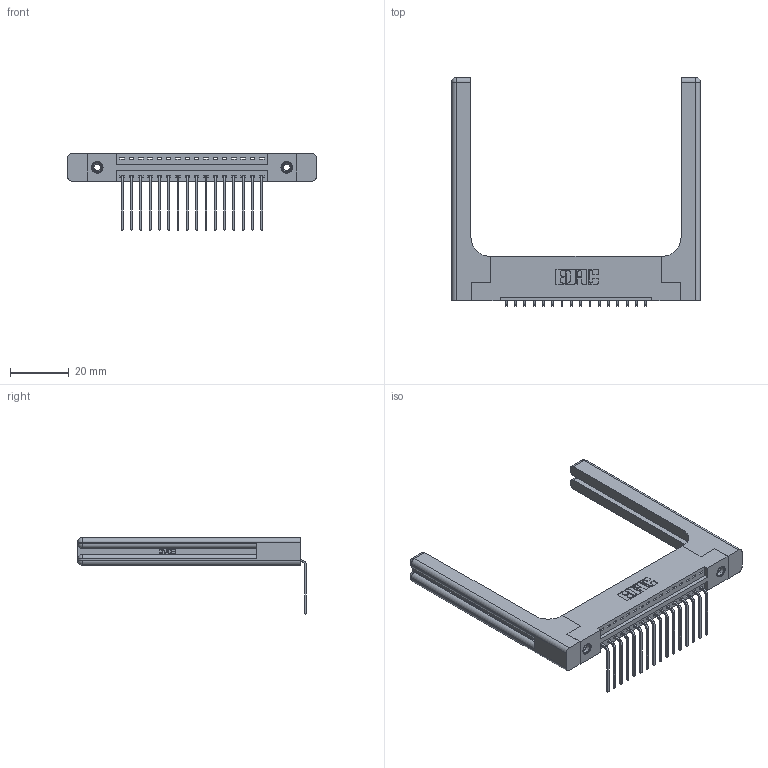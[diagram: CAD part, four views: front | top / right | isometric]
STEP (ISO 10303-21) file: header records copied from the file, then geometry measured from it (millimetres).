
FILE_DESCRIPTION (( 'STEP AP203' ), '1' );
FILE_NAME ('346-016-559-158.STEP', '2022-05-05T11:11:57', ( '' ), ( '' ), 'SwSTEP 2.0', 'SolidWorks 2020', '' );
FILE_SCHEMA (( 'CONFIG_CONTROL_DESIGN' ));
Length unit declared in the file: inch
Products named in the file (5): 346-220-058_345-220-058; 345-250-001_345-250-001-102; 345-292-001_558 559 Tail - 1; 346-016-559-158; 346 Part_Flush Mounting Lugs - 0.156 Dia-TH
Assembly tree (21 placements, depth 2):
  346-016-559-158
    346 Part_Flush Mounting Lugs - 0.156 Dia-TH
    345-292-001_558 559 Tail - 1  x16
    345-250-001_345-250-001-102  x2
    346-220-058_345-220-058  x2
Bounding box: 84.86 x 78.04 x 26.16 mm (x, y, z)
Volume: 15497.6 mm3; surface area: 15212.2 mm2
Topology: 21 solids, 21 shells, 1352 faces, 3943 edges, 2586 vertices
Faces by surface type: plane 910, cylinder 382, bspline 36, cone 12, sphere 8, torus 4
Entity records: 19112 total; most frequent: CARTESIAN_POINT 4267, ORIENTED_EDGE 3012, DIRECTION 2726, EDGE_CURVE 1506, VECTOR 1218, LINE 1218, VERTEX_POINT 994, AXIS2_PLACEMENT_3D 754
